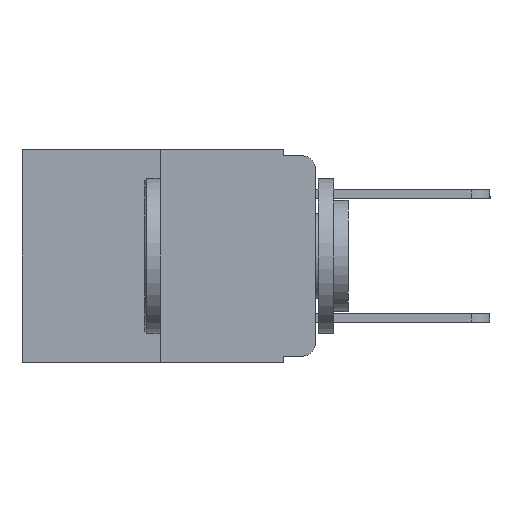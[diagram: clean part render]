
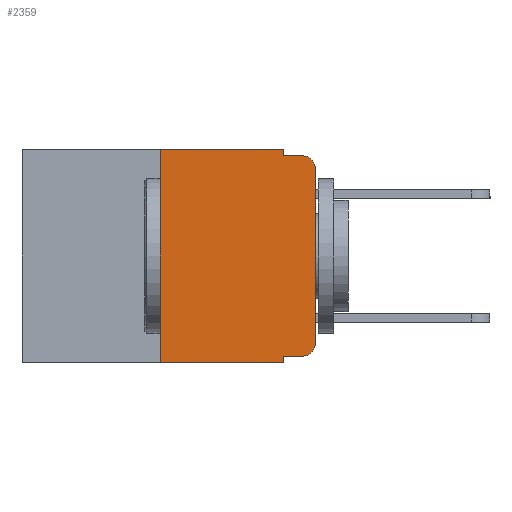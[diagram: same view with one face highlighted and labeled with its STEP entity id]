
A CAD part, left-side view. The second image highlights one B-rep face of the part: STEP entity #2359.
In plain terms, the highlighted planar face has unit normal (-1, 0, 0).
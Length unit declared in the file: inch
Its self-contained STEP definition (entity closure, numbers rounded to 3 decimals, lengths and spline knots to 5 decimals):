
#216 = VERTEX_POINT ( 'NONE', #14249 ) ;
#827 = LINE ( 'NONE', #11634, #5859 ) ;
#1227 = DIRECTION ( 'NONE',  ( -1., 0., 0. ) ) ;
#1536 = VERTEX_POINT ( 'NONE', #14493 ) ;
#1713 = VERTEX_POINT ( 'NONE', #11424 ) ;
#2359 = ADVANCED_FACE ( 'NONE', ( #18178 ), #6196, .F. ) ;
#2736 = EDGE_CURVE ( 'NONE', #20689, #15861, #17277, .T. ) ;
#2842 = CARTESIAN_POINT ( 'NONE',  ( 0., 0., -0.313 ) ) ;
#2988 = AXIS2_PLACEMENT_3D ( 'NONE', #11867, #1227, #13389 ) ;
#3528 = CARTESIAN_POINT ( 'NONE',  ( 0., 0.25, -0.343 ) ) ;
#3548 = DIRECTION ( 'NONE',  ( 0., 0., 1. ) ) ;
#4147 = LINE ( 'NONE', #12205, #16690 ) ;
#4561 = VERTEX_POINT ( 'NONE', #2842 ) ;
#4739 = EDGE_CURVE ( 'NONE', #12112, #19065, #13138, .T. ) ;
#4935 = CARTESIAN_POINT ( 'NONE',  ( 0., 0.473, -0.343 ) ) ;
#5307 = DIRECTION ( 'NONE',  ( 0., 0., -1. ) ) ;
#5621 = VERTEX_POINT ( 'NONE', #15173 ) ;
#5770 = DIRECTION ( 'NONE',  ( 0., -1., 0. ) ) ;
#5859 = VECTOR ( 'NONE', #18981, 39.37008 ) ;
#6152 = EDGE_CURVE ( 'NONE', #11959, #5621, #17452, .T. ) ;
#6196 = PLANE ( 'NONE',  #13673 ) ;
#6218 = DIRECTION ( 'NONE',  ( 1., 0., 0. ) ) ;
#7141 = DIRECTION ( 'NONE',  ( 0., 0., -1. ) ) ;
#7144 = DIRECTION ( 'NONE',  ( -1., 0., 0. ) ) ;
#7445 = DIRECTION ( 'NONE',  ( 0., -1., 0. ) ) ;
#8549 = VECTOR ( 'NONE', #7445, 39.37008 ) ;
#8804 = VECTOR ( 'NONE', #18848, 39.37008 ) ;
#8828 = VECTOR ( 'NONE', #7141, 39.37008 ) ;
#8945 = VECTOR ( 'NONE', #15259, 39.37008 ) ;
#9381 = LINE ( 'NONE', #17423, #8804 ) ;
#9522 = CIRCLE ( 'NONE', #19968, 0.02 ) ;
#9703 = EDGE_CURVE ( 'NONE', #20689, #12112, #4147, .T. ) ;
#9848 = CARTESIAN_POINT ( 'NONE',  ( 0., 0.051, -0.343 ) ) ;
#9947 = EDGE_LOOP ( 'NONE', ( #15450, #15665, #15729, #15860, #15879, #15956, #16113, #16767, #17656, #17727 ) ) ;
#10395 = EDGE_CURVE ( 'NONE', #1536, #4561, #9522, .T. ) ;
#10700 = VECTOR ( 'NONE', #16665, 39.37008 ) ;
#11183 = LINE ( 'NONE', #12164, #10700 ) ;
#11424 = CARTESIAN_POINT ( 'NONE',  ( 0., 0.051, -0.333 ) ) ;
#11634 = CARTESIAN_POINT ( 'NONE',  ( 0., 0.051, 0. ) ) ;
#11867 = CARTESIAN_POINT ( 'NONE',  ( 0., 0.02, -0.03 ) ) ;
#11959 = VERTEX_POINT ( 'NONE', #19052 ) ;
#12112 = VERTEX_POINT ( 'NONE', #16327 ) ;
#12164 = CARTESIAN_POINT ( 'NONE',  ( 0., 0.051, -0.01 ) ) ;
#12205 = CARTESIAN_POINT ( 'NONE',  ( 0., 0.25, 0. ) ) ;
#12406 = VECTOR ( 'NONE', #5770, 39.37008 ) ;
#12845 = EDGE_CURVE ( 'NONE', #19065, #216, #827, .T. ) ;
#12851 = LINE ( 'NONE', #15440, #8549 ) ;
#13138 = LINE ( 'NONE', #16874, #8945 ) ;
#13389 = DIRECTION ( 'NONE',  ( 0., 0., -1. ) ) ;
#13673 = AXIS2_PLACEMENT_3D ( 'NONE', #19069, #6218, #5307 ) ;
#14239 = EDGE_CURVE ( 'NONE', #216, #5621, #11183, .T. ) ;
#14249 = CARTESIAN_POINT ( 'NONE',  ( 0., 0.051, -0.01 ) ) ;
#14493 = CARTESIAN_POINT ( 'NONE',  ( 0., 0.02, -0.333 ) ) ;
#15173 = CARTESIAN_POINT ( 'NONE',  ( 0., 0.02, -0.01 ) ) ;
#15189 = CARTESIAN_POINT ( 'NONE',  ( 0., 0.051, 0. ) ) ;
#15259 = DIRECTION ( 'NONE',  ( 0., -1., 0. ) ) ;
#15440 = CARTESIAN_POINT ( 'NONE',  ( 0., 0.051, -0.333 ) ) ;
#15450 = ORIENTED_EDGE ( 'NONE', *, *, #21102, .T. ) ;
#15665 = ORIENTED_EDGE ( 'NONE', *, *, #6152, .T. ) ;
#15729 = ORIENTED_EDGE ( 'NONE', *, *, #14239, .F. ) ;
#15860 = ORIENTED_EDGE ( 'NONE', *, *, #12845, .F. ) ;
#15861 = VERTEX_POINT ( 'NONE', #9848 ) ;
#15879 = ORIENTED_EDGE ( 'NONE', *, *, #4739, .F. ) ;
#15956 = ORIENTED_EDGE ( 'NONE', *, *, #9703, .F. ) ;
#16113 = ORIENTED_EDGE ( 'NONE', *, *, #2736, .T. ) ;
#16327 = CARTESIAN_POINT ( 'NONE',  ( 0., 0.25, 0. ) ) ;
#16567 = LINE ( 'NONE', #15189, #8828 ) ;
#16634 = CARTESIAN_POINT ( 'NONE',  ( 0., 0.02, -0.313 ) ) ;
#16665 = DIRECTION ( 'NONE',  ( 0., -1., 0. ) ) ;
#16690 = VECTOR ( 'NONE', #3548, 39.37008 ) ;
#16767 = ORIENTED_EDGE ( 'NONE', *, *, #20645, .F. ) ;
#16874 = CARTESIAN_POINT ( 'NONE',  ( 0., 0.473, 0. ) ) ;
#17077 = CARTESIAN_POINT ( 'NONE',  ( 0., 0.051, 0. ) ) ;
#17277 = LINE ( 'NONE', #4935, #12406 ) ;
#17423 = CARTESIAN_POINT ( 'NONE',  ( 0., 0., 0. ) ) ;
#17452 = CIRCLE ( 'NONE', #2988, 0.02 ) ;
#17656 = ORIENTED_EDGE ( 'NONE', *, *, #19699, .T. ) ;
#17727 = ORIENTED_EDGE ( 'NONE', *, *, #10395, .T. ) ;
#18048 = DIRECTION ( 'NONE',  ( 0., 0., -1. ) ) ;
#18178 = FACE_OUTER_BOUND ( 'NONE', #9947, .T. ) ;
#18848 = DIRECTION ( 'NONE',  ( 0., 0., 1. ) ) ;
#18981 = DIRECTION ( 'NONE',  ( 0., 0., -1. ) ) ;
#19052 = CARTESIAN_POINT ( 'NONE',  ( 0., 0., -0.03 ) ) ;
#19065 = VERTEX_POINT ( 'NONE', #17077 ) ;
#19069 = CARTESIAN_POINT ( 'NONE',  ( 0., 0.473, 0. ) ) ;
#19699 = EDGE_CURVE ( 'NONE', #1713, #1536, #12851, .T. ) ;
#19968 = AXIS2_PLACEMENT_3D ( 'NONE', #16634, #7144, #18048 ) ;
#20645 = EDGE_CURVE ( 'NONE', #1713, #15861, #16567, .T. ) ;
#20689 = VERTEX_POINT ( 'NONE', #3528 ) ;
#21102 = EDGE_CURVE ( 'NONE', #4561, #11959, #9381, .T. ) ;
